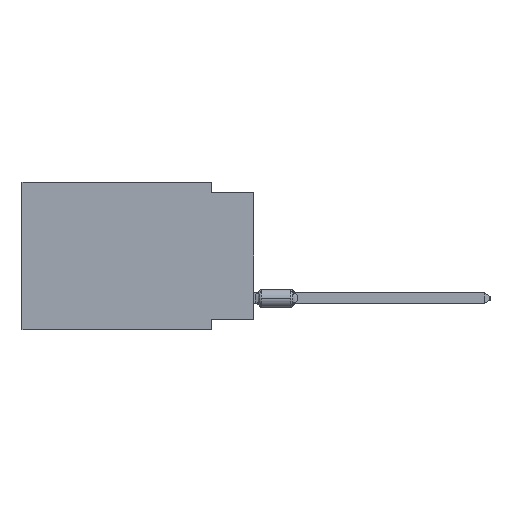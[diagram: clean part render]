
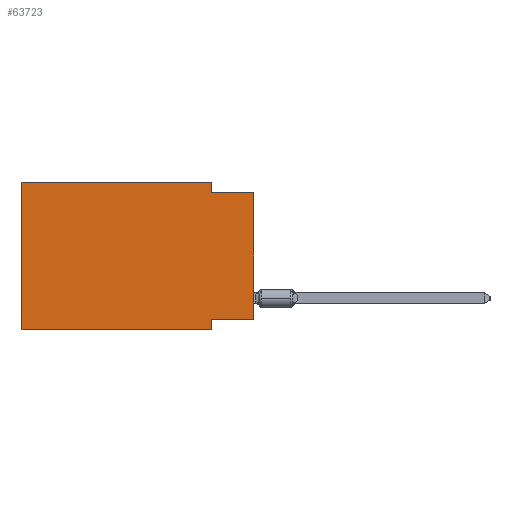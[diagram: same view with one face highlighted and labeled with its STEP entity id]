
A CAD part, left-side view. The second image highlights one B-rep face of the part: STEP entity #63723.
In plain terms, the highlighted planar face has unit normal (-1, 0, 0).
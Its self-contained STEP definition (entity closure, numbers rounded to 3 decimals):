
#1899 = ORIENTED_EDGE ( 'NONE', *, *, #72071, .F. ) ;
#2558 = EDGE_CURVE ( 'NONE', #16542, #39292, #5914, .T. ) ;
#2876 = VECTOR ( 'NONE', #51553, 1000. ) ;
#5914 = LINE ( 'NONE', #53338, #72746 ) ;
#6887 = EDGE_LOOP ( 'NONE', ( #59214, #33121, #48175, #43751, #10535, #48753, #69472, #1899 ) ) ;
#8803 = LINE ( 'NONE', #38346, #2876 ) ;
#9658 = CARTESIAN_POINT ( 'NONE',  ( 0., 0., 0. ) ) ;
#10535 = ORIENTED_EDGE ( 'NONE', *, *, #45603, .F. ) ;
#13260 = CARTESIAN_POINT ( 'NONE',  ( 0., 2.54, 0. ) ) ;
#15303 = EDGE_CURVE ( 'NONE', #26531, #54747, #45390, .T. ) ;
#15992 = DIRECTION ( 'NONE',  ( 0., 0., 1. ) ) ;
#16168 = VERTEX_POINT ( 'NONE', #44400 ) ;
#16542 = VERTEX_POINT ( 'NONE', #59795 ) ;
#18270 = CARTESIAN_POINT ( 'NONE',  ( 0., 0., -0.635 ) ) ;
#18627 = VERTEX_POINT ( 'NONE', #23369 ) ;
#19760 = EDGE_CURVE ( 'NONE', #18627, #54747, #54053, .T. ) ;
#21562 = LINE ( 'NONE', #76774, #70047 ) ;
#23369 = CARTESIAN_POINT ( 'NONE',  ( 0., 13.97, -8.89 ) ) ;
#24145 = VECTOR ( 'NONE', #41980, 1000. ) ;
#24426 = AXIS2_PLACEMENT_3D ( 'NONE', #63566, #34019, #28570 ) ;
#26531 = VERTEX_POINT ( 'NONE', #60457 ) ;
#28415 = LINE ( 'NONE', #40866, #56370 ) ;
#28570 = DIRECTION ( 'NONE',  ( 0., 0., -1. ) ) ;
#33121 = ORIENTED_EDGE ( 'NONE', *, *, #59630, .F. ) ;
#33714 = DIRECTION ( 'NONE',  ( 0., 0., -1. ) ) ;
#34019 = DIRECTION ( 'NONE',  ( 1., 0., 0. ) ) ;
#34414 = PLANE ( 'NONE',  #24426 ) ;
#34793 = FACE_OUTER_BOUND ( 'NONE', #6887, .T. ) ;
#38346 = CARTESIAN_POINT ( 'NONE',  ( 0., 2.54, 0. ) ) ;
#38794 = LINE ( 'NONE', #9658, #72428 ) ;
#39292 = VERTEX_POINT ( 'NONE', #13260 ) ;
#40866 = CARTESIAN_POINT ( 'NONE',  ( 0., 13.97, 0. ) ) ;
#41660 = DIRECTION ( 'NONE',  ( 0., -1., 0. ) ) ;
#41980 = DIRECTION ( 'NONE',  ( 0., -1., 0. ) ) ;
#43751 = ORIENTED_EDGE ( 'NONE', *, *, #2558, .F. ) ;
#44400 = CARTESIAN_POINT ( 'NONE',  ( 0., 2.54, -0.635 ) ) ;
#44613 = EDGE_CURVE ( 'NONE', #39292, #16168, #8803, .T. ) ;
#45390 = LINE ( 'NONE', #58217, #49894 ) ;
#45603 = EDGE_CURVE ( 'NONE', #18627, #16542, #28415, .T. ) ;
#48175 = ORIENTED_EDGE ( 'NONE', *, *, #44613, .F. ) ;
#48753 = ORIENTED_EDGE ( 'NONE', *, *, #19760, .T. ) ;
#49894 = VECTOR ( 'NONE', #33714, 1000. ) ;
#50874 = CARTESIAN_POINT ( 'NONE',  ( 0., 2.54, -8.89 ) ) ;
#51553 = DIRECTION ( 'NONE',  ( 0., 0., -1. ) ) ;
#53063 = DIRECTION ( 'NONE',  ( 0., 1., 0. ) ) ;
#53309 = CARTESIAN_POINT ( 'NONE',  ( 0., 13.97, -8.89 ) ) ;
#53338 = CARTESIAN_POINT ( 'NONE',  ( 0., 13.97, 0. ) ) ;
#53618 = VERTEX_POINT ( 'NONE', #73734 ) ;
#54053 = LINE ( 'NONE', #53309, #67734 ) ;
#54747 = VERTEX_POINT ( 'NONE', #50874 ) ;
#56370 = VECTOR ( 'NONE', #15992, 1000. ) ;
#58217 = CARTESIAN_POINT ( 'NONE',  ( 0., 2.54, -8.89 ) ) ;
#59214 = ORIENTED_EDGE ( 'NONE', *, *, #73217, .T. ) ;
#59630 = EDGE_CURVE ( 'NONE', #16168, #65760, #71537, .T. ) ;
#59795 = CARTESIAN_POINT ( 'NONE',  ( 0., 13.97, 0. ) ) ;
#60263 = DIRECTION ( 'NONE',  ( 0., -1., 0. ) ) ;
#60457 = CARTESIAN_POINT ( 'NONE',  ( 0., 2.54, -8.255 ) ) ;
#63566 = CARTESIAN_POINT ( 'NONE',  ( 0., 13.97, 0. ) ) ;
#63723 = ADVANCED_FACE ( 'NONE', ( #34793 ), #34414, .F. ) ;
#65760 = VERTEX_POINT ( 'NONE', #68853 ) ;
#67734 = VECTOR ( 'NONE', #60263, 1000. ) ;
#68853 = CARTESIAN_POINT ( 'NONE',  ( 0., 0., -0.635 ) ) ;
#69472 = ORIENTED_EDGE ( 'NONE', *, *, #15303, .F. ) ;
#70047 = VECTOR ( 'NONE', #53063, 1000. ) ;
#71537 = LINE ( 'NONE', #18270, #24145 ) ;
#72071 = EDGE_CURVE ( 'NONE', #53618, #26531, #21562, .T. ) ;
#72428 = VECTOR ( 'NONE', #73426, 1000. ) ;
#72746 = VECTOR ( 'NONE', #41660, 1000. ) ;
#73217 = EDGE_CURVE ( 'NONE', #53618, #65760, #38794, .T. ) ;
#73426 = DIRECTION ( 'NONE',  ( 0., 0., 1. ) ) ;
#73734 = CARTESIAN_POINT ( 'NONE',  ( 0., 0., -8.255 ) ) ;
#76774 = CARTESIAN_POINT ( 'NONE',  ( 0., 0., -8.255 ) ) ;
